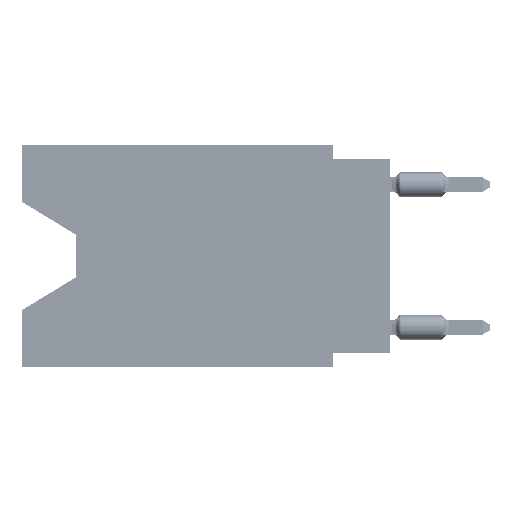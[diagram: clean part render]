
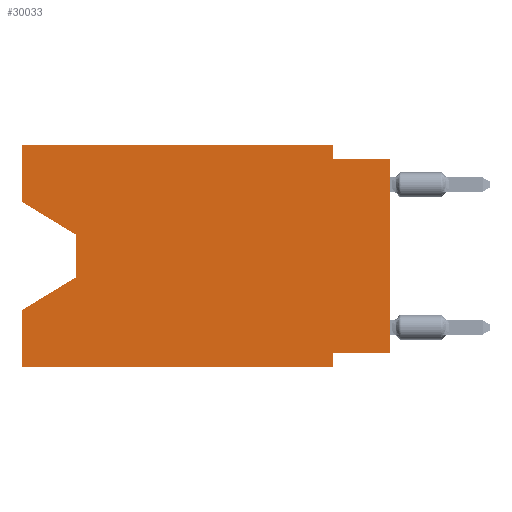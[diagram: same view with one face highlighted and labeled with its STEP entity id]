
A CAD part, left-side view. The second image highlights one B-rep face of the part: STEP entity #30033.
In plain terms, the highlighted planar face has unit normal (-1, 0, 0).
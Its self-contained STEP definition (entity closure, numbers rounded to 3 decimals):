
#82 = EDGE_CURVE ( 'NONE', #70162, #37211, #18784, .T. ) ;
#1363 = CARTESIAN_POINT ( 'NONE',  ( 0., 2.54, -9.906 ) ) ;
#1935 = ORIENTED_EDGE ( 'NONE', *, *, #61192, .T. ) ;
#2600 = DIRECTION ( 'NONE',  ( 0., 1., 0. ) ) ;
#2635 = LINE ( 'NONE', #53838, #47624 ) ;
#4829 = CARTESIAN_POINT ( 'NONE',  ( 0., 13.97, -5.893 ) ) ;
#4890 = ORIENTED_EDGE ( 'NONE', *, *, #47021, .F. ) ;
#4916 = EDGE_CURVE ( 'NONE', #52648, #25188, #2635, .T. ) ;
#5334 = LINE ( 'NONE', #7396, #52734 ) ;
#5850 = ORIENTED_EDGE ( 'NONE', *, *, #58091, .T. ) ;
#7396 = CARTESIAN_POINT ( 'NONE',  ( 0., 0., 0. ) ) ;
#7543 = LINE ( 'NONE', #11569, #62802 ) ;
#7598 = ORIENTED_EDGE ( 'NONE', *, *, #34875, .T. ) ;
#8589 = DIRECTION ( 'NONE',  ( 0., 0., -1. ) ) ;
#10197 = CARTESIAN_POINT ( 'NONE',  ( 0., 16.383, -2.546 ) ) ;
#10691 = VECTOR ( 'NONE', #8589, 1000. ) ;
#11254 = VECTOR ( 'NONE', #17323, 1000. ) ;
#11569 = CARTESIAN_POINT ( 'NONE',  ( 0., 0., -0.635 ) ) ;
#13050 = CARTESIAN_POINT ( 'NONE',  ( 0., 0., -0.635 ) ) ;
#13774 = CARTESIAN_POINT ( 'NONE',  ( 0., 16.383, -7.36 ) ) ;
#13913 = CARTESIAN_POINT ( 'NONE',  ( 0., 2.54, -9.906 ) ) ;
#14879 = ORIENTED_EDGE ( 'NONE', *, *, #58494, .F. ) ;
#16359 = ORIENTED_EDGE ( 'NONE', *, *, #30637, .F. ) ;
#16710 = CARTESIAN_POINT ( 'NONE',  ( 0., 16.383, -2.546 ) ) ;
#17323 = DIRECTION ( 'NONE',  ( 0., -1., 0. ) ) ;
#17939 = DIRECTION ( 'NONE',  ( 0., 0., 1. ) ) ;
#18784 = LINE ( 'NONE', #1363, #25004 ) ;
#22413 = VECTOR ( 'NONE', #43951, 1000. ) ;
#22868 = PLANE ( 'NONE',  #58245 ) ;
#24249 = ORIENTED_EDGE ( 'NONE', *, *, #82, .F. ) ;
#24766 = ORIENTED_EDGE ( 'NONE', *, *, #34367, .F. ) ;
#25004 = VECTOR ( 'NONE', #51501, 1000. ) ;
#25028 = CARTESIAN_POINT ( 'NONE',  ( 0., 2.54, -0.635 ) ) ;
#25188 = VERTEX_POINT ( 'NONE', #13774 ) ;
#30033 = ADVANCED_FACE ( 'NONE', ( #61048 ), #22868, .F. ) ;
#30212 = CARTESIAN_POINT ( 'NONE',  ( 0., 0., -9.271 ) ) ;
#30637 = EDGE_CURVE ( 'NONE', #58435, #34675, #47495, .T. ) ;
#33188 = ORIENTED_EDGE ( 'NONE', *, *, #61171, .F. ) ;
#33427 = DIRECTION ( 'NONE',  ( 0., 0., -1. ) ) ;
#33783 = VERTEX_POINT ( 'NONE', #39376 ) ;
#34367 = EDGE_CURVE ( 'NONE', #54246, #46432, #48343, .T. ) ;
#34675 = VERTEX_POINT ( 'NONE', #25028 ) ;
#34748 = CARTESIAN_POINT ( 'NONE',  ( 0., 16.383, 0. ) ) ;
#34875 = EDGE_CURVE ( 'NONE', #33783, #49940, #5334, .T. ) ;
#35072 = EDGE_LOOP ( 'NONE', ( #52416, #5850, #46886, #14879, #1935, #24249, #33188, #7598, #52669, #16359, #4890, #24766 ) ) ;
#36740 = DIRECTION ( 'NONE',  ( 0., 0.855, -0.519 ) ) ;
#36781 = EDGE_CURVE ( 'NONE', #34675, #49940, #7543, .T. ) ;
#37211 = VERTEX_POINT ( 'NONE', #13913 ) ;
#39376 = CARTESIAN_POINT ( 'NONE',  ( 0., 0., -9.271 ) ) ;
#39514 = VERTEX_POINT ( 'NONE', #50057 ) ;
#40836 = VECTOR ( 'NONE', #58588, 1000. ) ;
#40887 = VECTOR ( 'NONE', #42469, 1000. ) ;
#42469 = DIRECTION ( 'NONE',  ( 0., 0., 1. ) ) ;
#42901 = DIRECTION ( 'NONE',  ( 0., -0.855, -0.519 ) ) ;
#43951 = DIRECTION ( 'NONE',  ( 0., -1., 0. ) ) ;
#44460 = VECTOR ( 'NONE', #2600, 1000. ) ;
#44930 = LINE ( 'NONE', #34748, #11254 ) ;
#46432 = VERTEX_POINT ( 'NONE', #66844 ) ;
#46886 = ORIENTED_EDGE ( 'NONE', *, *, #4916, .T. ) ;
#47021 = EDGE_CURVE ( 'NONE', #46432, #58435, #44930, .T. ) ;
#47495 = LINE ( 'NONE', #52939, #10691 ) ;
#47624 = VECTOR ( 'NONE', #36740, 1000. ) ;
#48053 = VECTOR ( 'NONE', #71590, 1000. ) ;
#48343 = LINE ( 'NONE', #71245, #48053 ) ;
#48385 = LINE ( 'NONE', #70559, #40836 ) ;
#48734 = LINE ( 'NONE', #16710, #66114 ) ;
#49748 = EDGE_CURVE ( 'NONE', #54246, #60632, #48734, .T. ) ;
#49940 = VERTEX_POINT ( 'NONE', #13050 ) ;
#50054 = CARTESIAN_POINT ( 'NONE',  ( 0., 13.97, -4.013 ) ) ;
#50057 = CARTESIAN_POINT ( 'NONE',  ( 0., 16.383, -9.906 ) ) ;
#50167 = CARTESIAN_POINT ( 'NONE',  ( 0., 16.383, 0. ) ) ;
#50469 = DIRECTION ( 'NONE',  ( 0., -1., 0. ) ) ;
#51501 = DIRECTION ( 'NONE',  ( 0., 0., -1. ) ) ;
#52011 = LINE ( 'NONE', #30212, #44460 ) ;
#52416 = ORIENTED_EDGE ( 'NONE', *, *, #49748, .T. ) ;
#52648 = VERTEX_POINT ( 'NONE', #4829 ) ;
#52669 = ORIENTED_EDGE ( 'NONE', *, *, #36781, .F. ) ;
#52734 = VECTOR ( 'NONE', #17939, 1000. ) ;
#52939 = CARTESIAN_POINT ( 'NONE',  ( 0., 2.54, 0. ) ) ;
#53415 = CARTESIAN_POINT ( 'NONE',  ( 0., 2.54, 0. ) ) ;
#53838 = CARTESIAN_POINT ( 'NONE',  ( 0., 13.97, -5.893 ) ) ;
#54246 = VERTEX_POINT ( 'NONE', #10197 ) ;
#54482 = LINE ( 'NONE', #70476, #40887 ) ;
#55226 = CARTESIAN_POINT ( 'NONE',  ( 0., 16.383, -9.906 ) ) ;
#58091 = EDGE_CURVE ( 'NONE', #60632, #52648, #48385, .T. ) ;
#58245 = AXIS2_PLACEMENT_3D ( 'NONE', #50167, #66863, #33427 ) ;
#58435 = VERTEX_POINT ( 'NONE', #53415 ) ;
#58494 = EDGE_CURVE ( 'NONE', #39514, #25188, #54482, .T. ) ;
#58588 = DIRECTION ( 'NONE',  ( 0., 0., -1. ) ) ;
#60632 = VERTEX_POINT ( 'NONE', #50054 ) ;
#61048 = FACE_OUTER_BOUND ( 'NONE', #35072, .T. ) ;
#61171 = EDGE_CURVE ( 'NONE', #33783, #70162, #52011, .T. ) ;
#61192 = EDGE_CURVE ( 'NONE', #39514, #37211, #70514, .T. ) ;
#61245 = CARTESIAN_POINT ( 'NONE',  ( 0., 2.54, -9.271 ) ) ;
#62802 = VECTOR ( 'NONE', #50469, 1000. ) ;
#66114 = VECTOR ( 'NONE', #42901, 1000. ) ;
#66844 = CARTESIAN_POINT ( 'NONE',  ( 0., 16.383, 0. ) ) ;
#66863 = DIRECTION ( 'NONE',  ( 1., 0., 0. ) ) ;
#70162 = VERTEX_POINT ( 'NONE', #61245 ) ;
#70476 = CARTESIAN_POINT ( 'NONE',  ( 0., 16.383, 0. ) ) ;
#70514 = LINE ( 'NONE', #55226, #22413 ) ;
#70559 = CARTESIAN_POINT ( 'NONE',  ( 0., 13.97, -4.013 ) ) ;
#71245 = CARTESIAN_POINT ( 'NONE',  ( 0., 16.383, 0. ) ) ;
#71590 = DIRECTION ( 'NONE',  ( 0., 0., 1. ) ) ;
